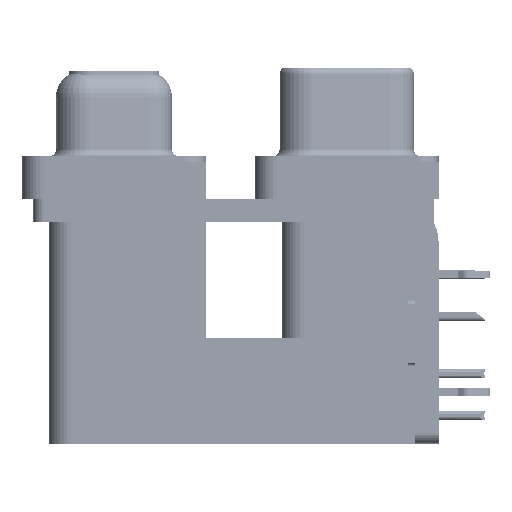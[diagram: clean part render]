
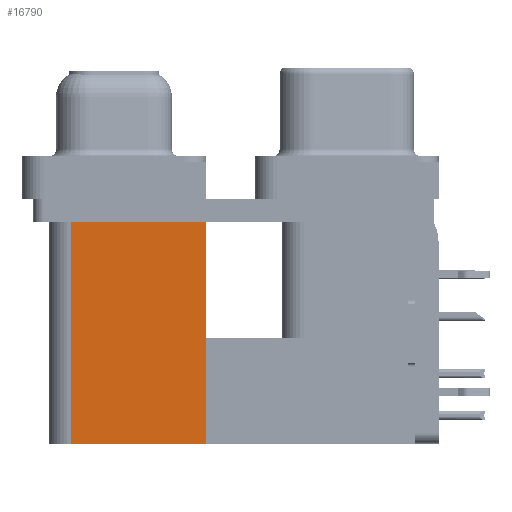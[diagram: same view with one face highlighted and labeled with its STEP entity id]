
A CAD part, left-side view. The second image highlights one B-rep face of the part: STEP entity #16790.
In plain terms, the highlighted planar face has unit normal (-1, 0, 0).
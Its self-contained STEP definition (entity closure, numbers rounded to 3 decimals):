
#771 = CARTESIAN_POINT ( 'NONE',  ( 3.79, 9.6, -19.2 ) ) ;
#1590 = VECTOR ( 'NONE', #4878, 1000. ) ;
#1762 = DIRECTION ( 'NONE',  ( 0., 1., 0. ) ) ;
#4878 = DIRECTION ( 'NONE',  ( 0., 0., 1. ) ) ;
#5708 = FACE_OUTER_BOUND ( 'NONE', #28661, .T. ) ;
#8643 = EDGE_CURVE ( 'NONE', #54624, #9057, #33192, .T. ) ;
#9057 = VERTEX_POINT ( 'NONE', #34783 ) ;
#13813 = CARTESIAN_POINT ( 'NONE',  ( 3.79, 18.8, -19.2 ) ) ;
#16055 = DIRECTION ( 'NONE',  ( 1., 0., 0. ) ) ;
#16790 = ADVANCED_FACE ( 'NONE', ( #5708 ), #21402, .F. ) ;
#16962 = VERTEX_POINT ( 'NONE', #18534 ) ;
#17274 = CARTESIAN_POINT ( 'NONE',  ( 3.79, 9.6, -19.2 ) ) ;
#18534 = CARTESIAN_POINT ( 'NONE',  ( 3.79, 18.8, -2.5 ) ) ;
#18579 = DIRECTION ( 'NONE',  ( 0., 1., 0. ) ) ;
#21014 = EDGE_CURVE ( 'NONE', #9057, #16962, #40859, .T. ) ;
#21402 = PLANE ( 'NONE',  #41465 ) ;
#22177 = ORIENTED_EDGE ( 'NONE', *, *, #21014, .F. ) ;
#27531 = EDGE_CURVE ( 'NONE', #67491, #16962, #44821, .T. ) ;
#28661 = EDGE_LOOP ( 'NONE', ( #32675, #22177, #46312, #66660 ) ) ;
#30647 = LINE ( 'NONE', #69941, #1590 ) ;
#32675 = ORIENTED_EDGE ( 'NONE', *, *, #27531, .T. ) ;
#33192 = LINE ( 'NONE', #771, #60009 ) ;
#34783 = CARTESIAN_POINT ( 'NONE',  ( 3.79, 18.8, -19.2 ) ) ;
#37872 = EDGE_CURVE ( 'NONE', #54624, #67491, #30647, .T. ) ;
#40859 = LINE ( 'NONE', #13813, #67880 ) ;
#41465 = AXIS2_PLACEMENT_3D ( 'NONE', #43093, #16055, #59413 ) ;
#43093 = CARTESIAN_POINT ( 'NONE',  ( 3.79, 9.6, -19.2 ) ) ;
#44821 = LINE ( 'NONE', #46227, #59219 ) ;
#46227 = CARTESIAN_POINT ( 'NONE',  ( 3.79, 9.6, -2.5 ) ) ;
#46312 = ORIENTED_EDGE ( 'NONE', *, *, #8643, .F. ) ;
#54624 = VERTEX_POINT ( 'NONE', #17274 ) ;
#59219 = VECTOR ( 'NONE', #1762, 1000. ) ;
#59413 = DIRECTION ( 'NONE',  ( 0., 1., 0. ) ) ;
#60009 = VECTOR ( 'NONE', #18579, 1000. ) ;
#61090 = CARTESIAN_POINT ( 'NONE',  ( 3.79, 9.6, -2.5 ) ) ;
#62862 = DIRECTION ( 'NONE',  ( 0., 0., 1. ) ) ;
#66660 = ORIENTED_EDGE ( 'NONE', *, *, #37872, .T. ) ;
#67491 = VERTEX_POINT ( 'NONE', #61090 ) ;
#67880 = VECTOR ( 'NONE', #62862, 1000. ) ;
#69941 = CARTESIAN_POINT ( 'NONE',  ( 3.79, 9.6, -19.2 ) ) ;
